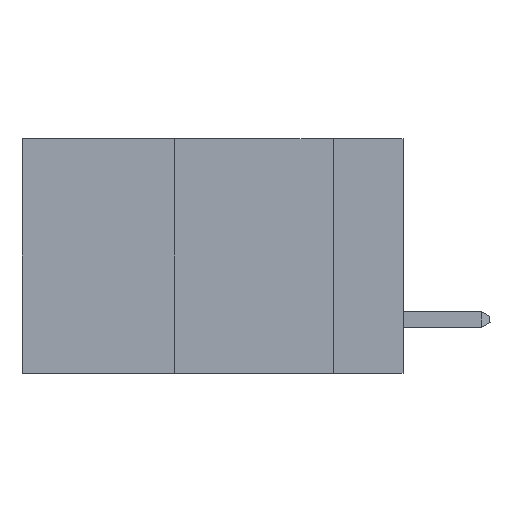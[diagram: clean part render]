
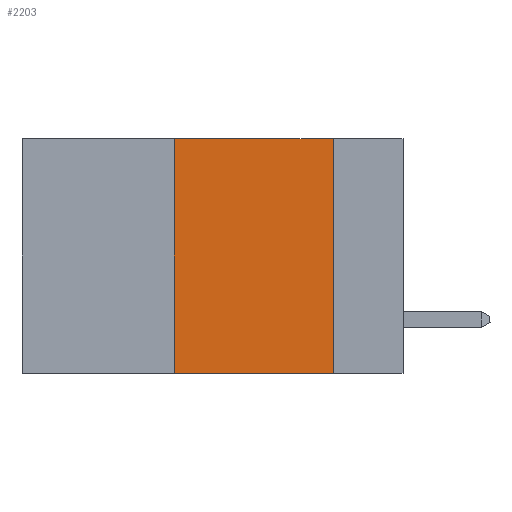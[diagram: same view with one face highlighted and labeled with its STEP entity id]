
A CAD part, left-side view. The second image highlights one B-rep face of the part: STEP entity #2203.
In plain terms, the highlighted planar face has unit normal (-1, 0, 0).
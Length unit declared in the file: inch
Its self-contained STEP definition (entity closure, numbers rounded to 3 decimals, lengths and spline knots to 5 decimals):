
#147 = VERTEX_POINT ( 'NONE', #4442 ) ;
#308 = CARTESIAN_POINT ( 'NONE',  ( 0., 0.11, 0. ) ) ;
#775 = CARTESIAN_POINT ( 'NONE',  ( 0., 0.36, 0. ) ) ;
#828 = CARTESIAN_POINT ( 'NONE',  ( 0., 0.6, 0. ) ) ;
#1471 = EDGE_CURVE ( 'NONE', #10736, #3809, #7815, .T. ) ;
#1734 = CARTESIAN_POINT ( 'NONE',  ( 0., 0.36, -0.37 ) ) ;
#2203 = ADVANCED_FACE ( 'NONE', ( #7628 ), #11970, .F. ) ;
#2969 = ORIENTED_EDGE ( 'NONE', *, *, #1471, .F. ) ;
#3148 = EDGE_LOOP ( 'NONE', ( #2969, #11164, #3303, #8392 ) ) ;
#3303 = ORIENTED_EDGE ( 'NONE', *, *, #5747, .F. ) ;
#3420 = VECTOR ( 'NONE', #3613, 39.37008 ) ;
#3613 = DIRECTION ( 'NONE',  ( 0., -1., 0. ) ) ;
#3809 = VERTEX_POINT ( 'NONE', #9902 ) ;
#4067 = AXIS2_PLACEMENT_3D ( 'NONE', #828, #9163, #6469 ) ;
#4442 = CARTESIAN_POINT ( 'NONE',  ( 0., 0.36, 0. ) ) ;
#4467 = LINE ( 'NONE', #10115, #3420 ) ;
#5271 = EDGE_CURVE ( 'NONE', #9758, #3809, #9846, .T. ) ;
#5526 = DIRECTION ( 'NONE',  ( 0., 0., -1. ) ) ;
#5747 = EDGE_CURVE ( 'NONE', #9758, #147, #6228, .T. ) ;
#6228 = LINE ( 'NONE', #775, #10805 ) ;
#6469 = DIRECTION ( 'NONE',  ( 0., 0., -1. ) ) ;
#6587 = CARTESIAN_POINT ( 'NONE',  ( 0., 0.6, -0.37 ) ) ;
#7233 = EDGE_CURVE ( 'NONE', #147, #10736, #4467, .T. ) ;
#7628 = FACE_OUTER_BOUND ( 'NONE', #3148, .T. ) ;
#7815 = LINE ( 'NONE', #11011, #8983 ) ;
#8186 = DIRECTION ( 'NONE',  ( 0., 0., 1. ) ) ;
#8392 = ORIENTED_EDGE ( 'NONE', *, *, #5271, .T. ) ;
#8983 = VECTOR ( 'NONE', #5526, 39.37008 ) ;
#9163 = DIRECTION ( 'NONE',  ( 1., 0., 0. ) ) ;
#9386 = VECTOR ( 'NONE', #9482, 39.37008 ) ;
#9482 = DIRECTION ( 'NONE',  ( 0., -1., 0. ) ) ;
#9758 = VERTEX_POINT ( 'NONE', #1734 ) ;
#9846 = LINE ( 'NONE', #6587, #9386 ) ;
#9902 = CARTESIAN_POINT ( 'NONE',  ( 0., 0.11, -0.37 ) ) ;
#10115 = CARTESIAN_POINT ( 'NONE',  ( 0., 0.6, 0. ) ) ;
#10736 = VERTEX_POINT ( 'NONE', #308 ) ;
#10805 = VECTOR ( 'NONE', #8186, 39.37008 ) ;
#11011 = CARTESIAN_POINT ( 'NONE',  ( 0., 0.11, 0. ) ) ;
#11164 = ORIENTED_EDGE ( 'NONE', *, *, #7233, .F. ) ;
#11970 = PLANE ( 'NONE',  #4067 ) ;
